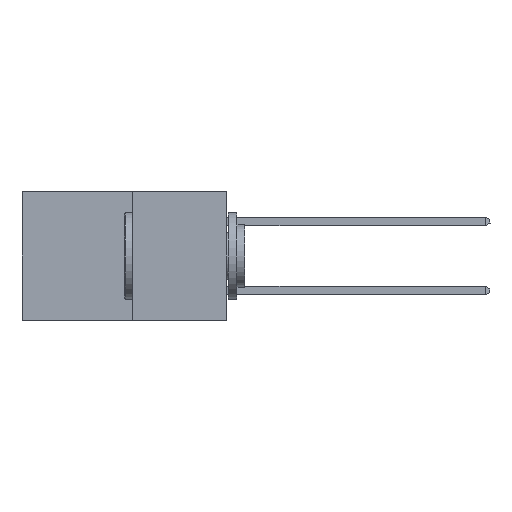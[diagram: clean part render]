
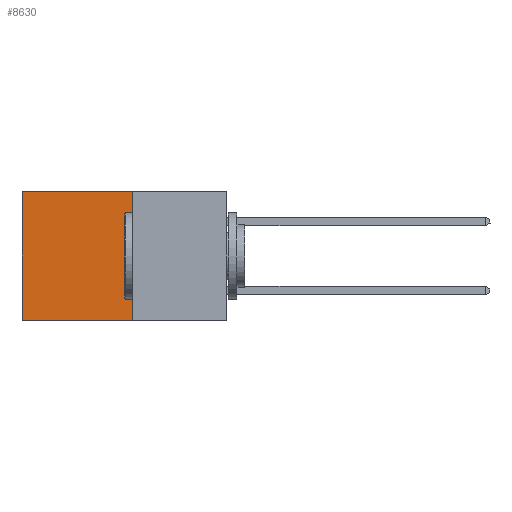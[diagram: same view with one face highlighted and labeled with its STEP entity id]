
A CAD part, left-side view. The second image highlights one B-rep face of the part: STEP entity #8630.
In plain terms, the highlighted planar face has unit normal (-1, 0, 0).
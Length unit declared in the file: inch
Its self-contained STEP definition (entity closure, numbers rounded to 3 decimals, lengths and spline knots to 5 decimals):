
#56 = ORIENTED_EDGE ( 'NONE', *, *, #16118, .T. ) ;
#219 = ORIENTED_EDGE ( 'NONE', *, *, #10620, .F. ) ;
#781 = CARTESIAN_POINT ( 'NONE',  ( 0.277, 0.27, -0.37 ) ) ;
#951 = ORIENTED_EDGE ( 'NONE', *, *, #11652, .F. ) ;
#1078 = ORIENTED_EDGE ( 'NONE', *, *, #10683, .T. ) ;
#1876 = DIRECTION ( 'NONE',  ( 0., 1., 0. ) ) ;
#3391 = LINE ( 'NONE', #7577, #7075 ) ;
#3681 = CARTESIAN_POINT ( 'NONE',  ( 0.277, 0.27, -0.37 ) ) ;
#3793 = CARTESIAN_POINT ( 'NONE',  ( 0.277, 0.27, -0.37 ) ) ;
#4368 = VERTEX_POINT ( 'NONE', #3793 ) ;
#4917 = DIRECTION ( 'NONE',  ( 0., 1., 0. ) ) ;
#5303 = DIRECTION ( 'NONE',  ( 1., 0., 0. ) ) ;
#7075 = VECTOR ( 'NONE', #17130, 39.37008 ) ;
#7095 = CARTESIAN_POINT ( 'NONE',  ( 0.277, 0.59, 0. ) ) ;
#7493 = CARTESIAN_POINT ( 'NONE',  ( 0.277, 0.27, -0.37 ) ) ;
#7577 = CARTESIAN_POINT ( 'NONE',  ( 0.277, 0.59, -0.37 ) ) ;
#7680 = CARTESIAN_POINT ( 'NONE',  ( 0.277, 0.27, 0. ) ) ;
#7769 = VECTOR ( 'NONE', #10614, 39.37008 ) ;
#8630 = ADVANCED_FACE ( 'NONE', ( #17033 ), #13673, .F. ) ;
#8920 = LINE ( 'NONE', #7680, #12657 ) ;
#9492 = CARTESIAN_POINT ( 'NONE',  ( 0.277, 0.27, 0. ) ) ;
#10182 = VERTEX_POINT ( 'NONE', #9492 ) ;
#10614 = DIRECTION ( 'NONE',  ( 0., 0., -1. ) ) ;
#10620 = EDGE_CURVE ( 'NONE', #4368, #14524, #13539, .T. ) ;
#10683 = EDGE_CURVE ( 'NONE', #10182, #16607, #8920, .T. ) ;
#11652 = EDGE_CURVE ( 'NONE', #10182, #4368, #15182, .T. ) ;
#12657 = VECTOR ( 'NONE', #4917, 39.37008 ) ;
#13539 = LINE ( 'NONE', #7493, #16603 ) ;
#13673 = PLANE ( 'NONE',  #16367 ) ;
#14524 = VERTEX_POINT ( 'NONE', #15714 ) ;
#15022 = DIRECTION ( 'NONE',  ( 0., 0., -1. ) ) ;
#15182 = LINE ( 'NONE', #3681, #7769 ) ;
#15714 = CARTESIAN_POINT ( 'NONE',  ( 0.277, 0.59, -0.37 ) ) ;
#16118 = EDGE_CURVE ( 'NONE', #16607, #14524, #3391, .T. ) ;
#16367 = AXIS2_PLACEMENT_3D ( 'NONE', #781, #5303, #15022 ) ;
#16603 = VECTOR ( 'NONE', #1876, 39.37008 ) ;
#16607 = VERTEX_POINT ( 'NONE', #7095 ) ;
#17033 = FACE_OUTER_BOUND ( 'NONE', #17368, .T. ) ;
#17130 = DIRECTION ( 'NONE',  ( 0., 0., -1. ) ) ;
#17368 = EDGE_LOOP ( 'NONE', ( #56, #219, #951, #1078 ) ) ;
